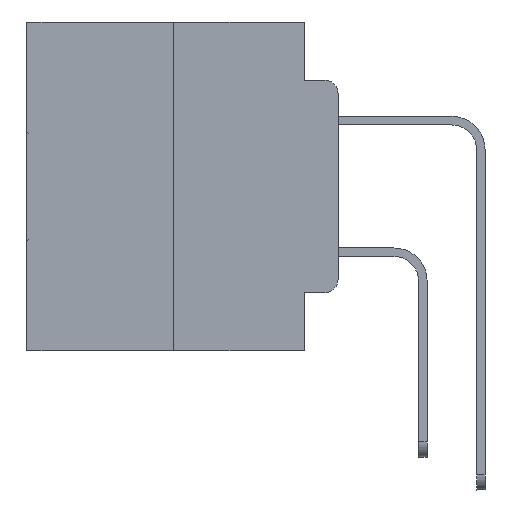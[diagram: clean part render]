
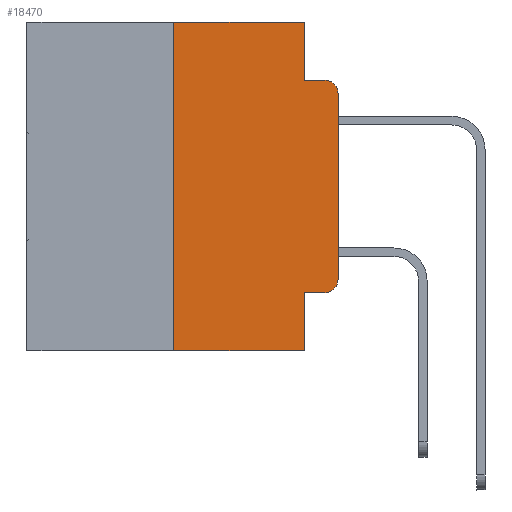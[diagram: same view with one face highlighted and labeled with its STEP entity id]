
A CAD part, left-side view. The second image highlights one B-rep face of the part: STEP entity #18470.
In plain terms, the highlighted planar face has unit normal (-1, 0, 0).
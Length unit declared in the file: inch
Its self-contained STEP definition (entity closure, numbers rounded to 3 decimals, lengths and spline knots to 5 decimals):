
#260 = PLANE ( 'NONE',  #23164 ) ;
#779 = DIRECTION ( 'NONE',  ( 0., 0., -1. ) ) ;
#905 = CARTESIAN_POINT ( 'NONE',  ( 0., 0.25, 0. ) ) ;
#977 = DIRECTION ( 'NONE',  ( 0., 0., 1. ) ) ;
#1635 = VECTOR ( 'NONE', #24439, 39.37008 ) ;
#1901 = CARTESIAN_POINT ( 'NONE',  ( 0., 0.051, 0. ) ) ;
#2467 = AXIS2_PLACEMENT_3D ( 'NONE', #29905, #15576, #779 ) ;
#2795 = DIRECTION ( 'NONE',  ( 1., 0., 0. ) ) ;
#2808 = VERTEX_POINT ( 'NONE', #905 ) ;
#3239 = CARTESIAN_POINT ( 'NONE',  ( 0., 0.051, 0. ) ) ;
#3369 = DIRECTION ( 'NONE',  ( 0., -1., 0. ) ) ;
#3640 = VECTOR ( 'NONE', #17758, 39.37008 ) ;
#4121 = EDGE_CURVE ( 'NONE', #20845, #26769, #7990, .T. ) ;
#4815 = CARTESIAN_POINT ( 'NONE',  ( 0., 0., -0.1085 ) ) ;
#5363 = ORIENTED_EDGE ( 'NONE', *, *, #4121, .T. ) ;
#5511 = VERTEX_POINT ( 'NONE', #26717 ) ;
#5757 = EDGE_CURVE ( 'NONE', #5511, #2808, #17496, .T. ) ;
#6185 = DIRECTION ( 'NONE',  ( 0., -1., 0. ) ) ;
#6716 = VECTOR ( 'NONE', #14938, 39.37008 ) ;
#7014 = ORIENTED_EDGE ( 'NONE', *, *, #20217, .T. ) ;
#7418 = EDGE_CURVE ( 'NONE', #23245, #23706, #10421, .T. ) ;
#7442 = CARTESIAN_POINT ( 'NONE',  ( 0., 0.473, -0.5 ) ) ;
#7602 = LINE ( 'NONE', #1901, #19812 ) ;
#7990 = CIRCLE ( 'NONE', #31452, 0.02 ) ;
#8203 = LINE ( 'NONE', #7442, #1635 ) ;
#8205 = CARTESIAN_POINT ( 'NONE',  ( 0., 0.473, 0. ) ) ;
#8218 = ORIENTED_EDGE ( 'NONE', *, *, #18900, .F. ) ;
#8588 = CARTESIAN_POINT ( 'NONE',  ( 0., 0.051, -0.5 ) ) ;
#9223 = DIRECTION ( 'NONE',  ( 0., 0., -1. ) ) ;
#9292 = ORIENTED_EDGE ( 'NONE', *, *, #27995, .F. ) ;
#10421 = LINE ( 'NONE', #18754, #28932 ) ;
#10853 = LINE ( 'NONE', #8205, #13169 ) ;
#11279 = CARTESIAN_POINT ( 'NONE',  ( 0., 0.051, -0.4115 ) ) ;
#12403 = CARTESIAN_POINT ( 'NONE',  ( 0., 0.051, -0.0885 ) ) ;
#12568 = FACE_OUTER_BOUND ( 'NONE', #14817, .T. ) ;
#13169 = VECTOR ( 'NONE', #3369, 39.37008 ) ;
#13938 = DIRECTION ( 'NONE',  ( 0., 0., -1. ) ) ;
#13970 = LINE ( 'NONE', #12403, #6716 ) ;
#14817 = EDGE_LOOP ( 'NONE', ( #18850, #5363, #17053, #31163, #9292, #18493, #7014, #8218, #17080, #21182 ) ) ;
#14938 = DIRECTION ( 'NONE',  ( 0., -1., 0. ) ) ;
#15429 = EDGE_CURVE ( 'NONE', #26925, #17163, #31214, .T. ) ;
#15576 = DIRECTION ( 'NONE',  ( -1., 0., 0. ) ) ;
#15862 = CARTESIAN_POINT ( 'NONE',  ( 0., 0.02, -0.0885 ) ) ;
#16000 = CARTESIAN_POINT ( 'NONE',  ( 0., 0.051, -0.4115 ) ) ;
#16367 = VERTEX_POINT ( 'NONE', #30489 ) ;
#17053 = ORIENTED_EDGE ( 'NONE', *, *, #25902, .F. ) ;
#17080 = ORIENTED_EDGE ( 'NONE', *, *, #15429, .T. ) ;
#17163 = VERTEX_POINT ( 'NONE', #19498 ) ;
#17496 = LINE ( 'NONE', #20869, #3640 ) ;
#17758 = DIRECTION ( 'NONE',  ( 0., 0., 1. ) ) ;
#18470 = ADVANCED_FACE ( 'NONE', ( #12568 ), #260, .F. ) ;
#18493 = ORIENTED_EDGE ( 'NONE', *, *, #5757, .F. ) ;
#18703 = VERTEX_POINT ( 'NONE', #8588 ) ;
#18754 = CARTESIAN_POINT ( 'NONE',  ( 0., 0.051, 0. ) ) ;
#18850 = ORIENTED_EDGE ( 'NONE', *, *, #22699, .T. ) ;
#18900 = EDGE_CURVE ( 'NONE', #26925, #18703, #7602, .T. ) ;
#19498 = CARTESIAN_POINT ( 'NONE',  ( 0., 0.02, -0.4115 ) ) ;
#19812 = VECTOR ( 'NONE', #9223, 39.37008 ) ;
#19813 = CARTESIAN_POINT ( 'NONE',  ( 0., 0.473, 0. ) ) ;
#19926 = DIRECTION ( 'NONE',  ( 0., 0., -1. ) ) ;
#20217 = EDGE_CURVE ( 'NONE', #5511, #18703, #8203, .T. ) ;
#20845 = VERTEX_POINT ( 'NONE', #4815 ) ;
#20869 = CARTESIAN_POINT ( 'NONE',  ( 0., 0.25, 0. ) ) ;
#21182 = ORIENTED_EDGE ( 'NONE', *, *, #26086, .T. ) ;
#22699 = EDGE_CURVE ( 'NONE', #16367, #20845, #31469, .T. ) ;
#22789 = CIRCLE ( 'NONE', #2467, 0.02 ) ;
#22897 = CARTESIAN_POINT ( 'NONE',  ( 0., 0., 0. ) ) ;
#23164 = AXIS2_PLACEMENT_3D ( 'NONE', #19813, #2795, #19926 ) ;
#23245 = VERTEX_POINT ( 'NONE', #3239 ) ;
#23706 = VERTEX_POINT ( 'NONE', #31357 ) ;
#24439 = DIRECTION ( 'NONE',  ( 0., -1., 0. ) ) ;
#24923 = DIRECTION ( 'NONE',  ( 0., 0., -1. ) ) ;
#24929 = DIRECTION ( 'NONE',  ( -1., 0., 0. ) ) ;
#25181 = VECTOR ( 'NONE', #977, 39.37008 ) ;
#25902 = EDGE_CURVE ( 'NONE', #23706, #26769, #13970, .T. ) ;
#26086 = EDGE_CURVE ( 'NONE', #17163, #16367, #22789, .T. ) ;
#26717 = CARTESIAN_POINT ( 'NONE',  ( 0., 0.25, -0.5 ) ) ;
#26769 = VERTEX_POINT ( 'NONE', #15862 ) ;
#26925 = VERTEX_POINT ( 'NONE', #11279 ) ;
#27734 = CARTESIAN_POINT ( 'NONE',  ( 0., 0.02, -0.1085 ) ) ;
#27995 = EDGE_CURVE ( 'NONE', #2808, #23245, #10853, .T. ) ;
#28251 = VECTOR ( 'NONE', #6185, 39.37008 ) ;
#28932 = VECTOR ( 'NONE', #13938, 39.37008 ) ;
#29905 = CARTESIAN_POINT ( 'NONE',  ( 0., 0.02, -0.3915 ) ) ;
#30489 = CARTESIAN_POINT ( 'NONE',  ( 0., 0., -0.3915 ) ) ;
#31163 = ORIENTED_EDGE ( 'NONE', *, *, #7418, .F. ) ;
#31214 = LINE ( 'NONE', #16000, #28251 ) ;
#31357 = CARTESIAN_POINT ( 'NONE',  ( 0., 0.051, -0.0885 ) ) ;
#31452 = AXIS2_PLACEMENT_3D ( 'NONE', #27734, #24929, #24923 ) ;
#31469 = LINE ( 'NONE', #22897, #25181 ) ;
